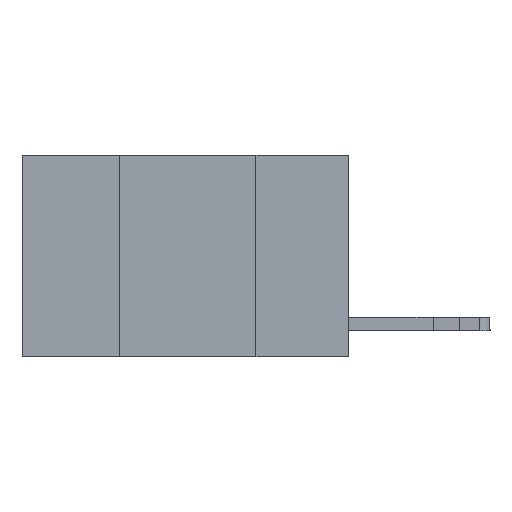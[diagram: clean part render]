
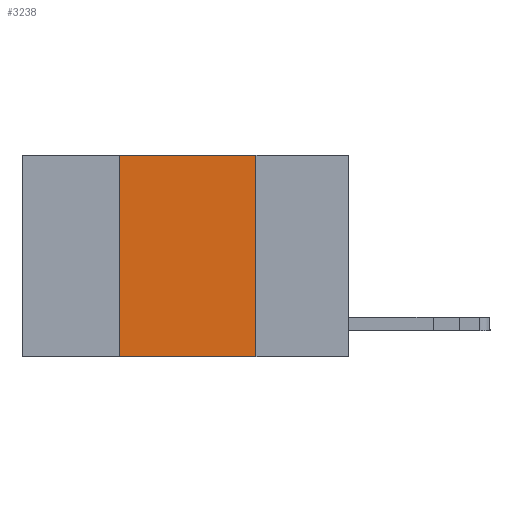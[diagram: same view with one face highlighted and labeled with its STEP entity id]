
A CAD part, left-side view. The second image highlights one B-rep face of the part: STEP entity #3238.
In plain terms, the highlighted planar face has unit normal (-1, 0, 0).
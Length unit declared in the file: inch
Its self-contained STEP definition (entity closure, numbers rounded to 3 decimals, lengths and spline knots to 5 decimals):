
#192 = ORIENTED_EDGE ( 'NONE', *, *, #4521, .F. ) ;
#594 = LINE ( 'NONE', #8525, #12267 ) ;
#901 = ORIENTED_EDGE ( 'NONE', *, *, #1953, .T. ) ;
#1043 = LINE ( 'NONE', #4911, #8528 ) ;
#1953 = EDGE_CURVE ( 'NONE', #5810, #12028, #14518, .T. ) ;
#2481 = DIRECTION ( 'NONE',  ( 0., -1., 0. ) ) ;
#2787 = VECTOR ( 'NONE', #3124, 39.37008 ) ;
#3124 = DIRECTION ( 'NONE',  ( 0., -1., 0. ) ) ;
#3238 = ADVANCED_FACE ( 'NONE', ( #9444 ), #9741, .F. ) ;
#3699 = DIRECTION ( 'NONE',  ( 0., 0., -1. ) ) ;
#4041 = AXIS2_PLACEMENT_3D ( 'NONE', #4908, #12904, #3699 ) ;
#4521 = EDGE_CURVE ( 'NONE', #5810, #11759, #1043, .T. ) ;
#4908 = CARTESIAN_POINT ( 'NONE',  ( 0., 0.6, 0. ) ) ;
#4911 = CARTESIAN_POINT ( 'NONE',  ( 0., 0.42, 0. ) ) ;
#5276 = CARTESIAN_POINT ( 'NONE',  ( 0., 0.17, 0. ) ) ;
#5810 = VERTEX_POINT ( 'NONE', #6537 ) ;
#6537 = CARTESIAN_POINT ( 'NONE',  ( 0., 0.42, -0.37 ) ) ;
#7692 = ORIENTED_EDGE ( 'NONE', *, *, #8061, .F. ) ;
#7770 = EDGE_LOOP ( 'NONE', ( #7692, #14166, #192, #901 ) ) ;
#8061 = EDGE_CURVE ( 'NONE', #9560, #12028, #594, .T. ) ;
#8145 = CARTESIAN_POINT ( 'NONE',  ( 0., 0.6, 0. ) ) ;
#8525 = CARTESIAN_POINT ( 'NONE',  ( 0., 0.17, 0. ) ) ;
#8528 = VECTOR ( 'NONE', #10731, 39.37008 ) ;
#8547 = CARTESIAN_POINT ( 'NONE',  ( 0., 0.17, -0.37 ) ) ;
#8934 = CARTESIAN_POINT ( 'NONE',  ( 0., 0.42, 0. ) ) ;
#9444 = FACE_OUTER_BOUND ( 'NONE', #7770, .T. ) ;
#9560 = VERTEX_POINT ( 'NONE', #5276 ) ;
#9741 = PLANE ( 'NONE',  #4041 ) ;
#10731 = DIRECTION ( 'NONE',  ( 0., 0., 1. ) ) ;
#11118 = EDGE_CURVE ( 'NONE', #11759, #9560, #12964, .T. ) ;
#11759 = VERTEX_POINT ( 'NONE', #8934 ) ;
#12028 = VERTEX_POINT ( 'NONE', #8547 ) ;
#12267 = VECTOR ( 'NONE', #13128, 39.37008 ) ;
#12904 = DIRECTION ( 'NONE',  ( 1., 0., 0. ) ) ;
#12964 = LINE ( 'NONE', #8145, #14000 ) ;
#13128 = DIRECTION ( 'NONE',  ( 0., 0., -1. ) ) ;
#13466 = CARTESIAN_POINT ( 'NONE',  ( 0., 0.6, -0.37 ) ) ;
#14000 = VECTOR ( 'NONE', #2481, 39.37008 ) ;
#14166 = ORIENTED_EDGE ( 'NONE', *, *, #11118, .F. ) ;
#14518 = LINE ( 'NONE', #13466, #2787 ) ;
